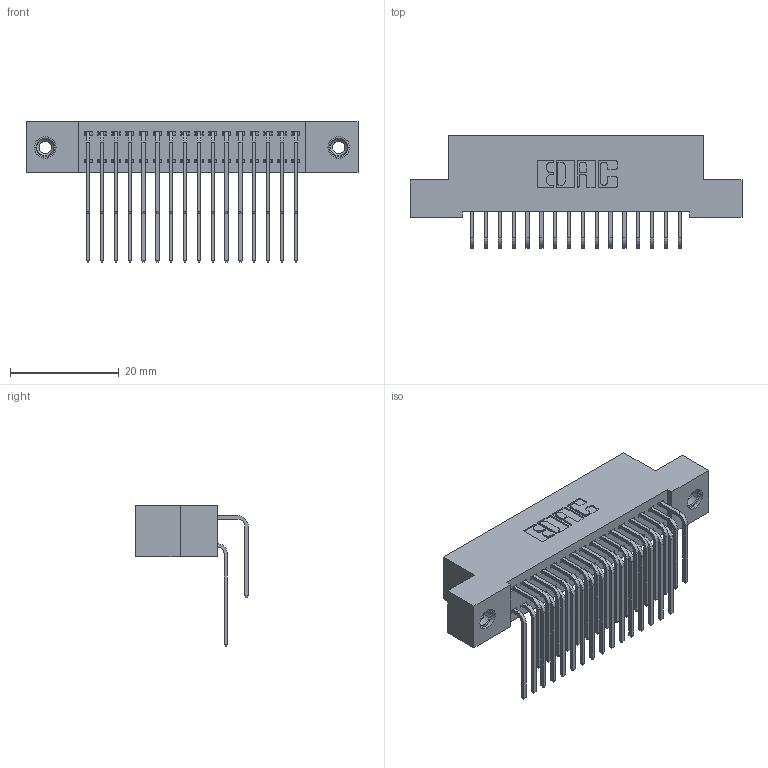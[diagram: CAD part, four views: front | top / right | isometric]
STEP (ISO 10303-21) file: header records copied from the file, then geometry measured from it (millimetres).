
FILE_DESCRIPTION (( 'STEP AP203' ), '1' );
FILE_NAME ('342-032-559-208.STEP', '2019-10-02T11:28:01', ( '' ), ( '' ), 'SwSTEP 2.0', 'SolidWorks 2016', '' );
FILE_SCHEMA (( 'CONFIG_CONTROL_DESIGN' ));
Length unit declared in the file: inch
Products named in the file (5): 342 Part_TI; 345-292-001_558 559 Tail - 1; 345-292-001_559 Tail - 2; 345-250-001_345-250-003-102; 342-032-559-208
Assembly tree (35 placements, depth 2):
  342-032-559-208
    342 Part_TI
    345-292-001_558 559 Tail - 1  x16
    345-292-001_559 Tail - 2  x16
    345-250-001_345-250-003-102  x2
Bounding box: 60.96 x 20.64 x 25.78 mm (x, y, z)
Volume: 5533.1 mm3; surface area: 9211.2 mm2
Topology: 35 solids, 35 shells, 1898 faces, 5587 edges, 3674 vertices
Faces by surface type: plane 1314, cylinder 568, cone 12, torus 4
Entity records: 16494 total; most frequent: CARTESIAN_POINT 2796, ORIENTED_EDGE 2674, DIRECTION 2447, EDGE_CURVE 1337, LINE 1149, VECTOR 1149, VERTEX_POINT 884, AXIS2_PLACEMENT_3D 649
